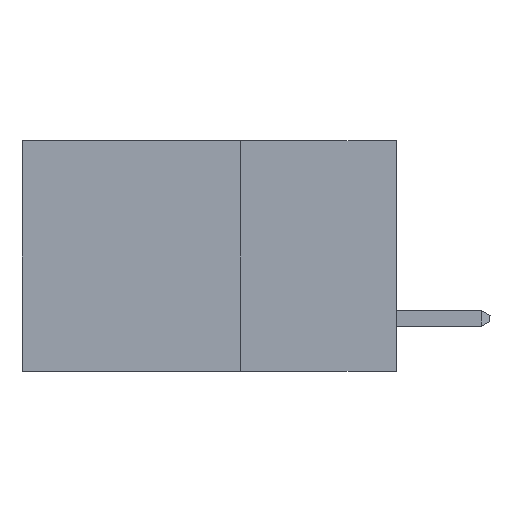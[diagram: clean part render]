
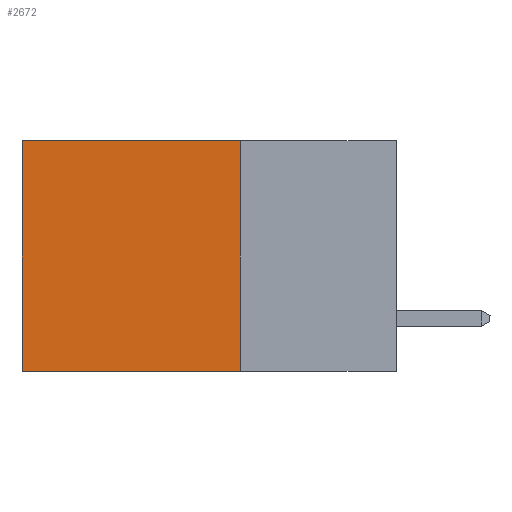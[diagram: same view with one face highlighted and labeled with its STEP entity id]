
A CAD part, left-side view. The second image highlights one B-rep face of the part: STEP entity #2672.
In plain terms, the highlighted planar face has unit normal (-1, 0, 0).
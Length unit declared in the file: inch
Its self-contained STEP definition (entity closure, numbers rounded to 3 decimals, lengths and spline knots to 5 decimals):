
#148 = EDGE_CURVE ( 'NONE', #840, #9183, #6486, .T. ) ;
#196 = CARTESIAN_POINT ( 'NONE',  ( 0.2615, 0.6, -0.37 ) ) ;
#212 = DIRECTION ( 'NONE',  ( 0., 0., -1. ) ) ;
#498 = EDGE_CURVE ( 'NONE', #6003, #9183, #7599, .T. ) ;
#619 = CARTESIAN_POINT ( 'NONE',  ( 0.2615, 0.25, 0. ) ) ;
#667 = EDGE_LOOP ( 'NONE', ( #7518, #4641, #7923, #6467 ) ) ;
#736 = CARTESIAN_POINT ( 'NONE',  ( 0.2615, 0.25, 0. ) ) ;
#840 = VERTEX_POINT ( 'NONE', #8633 ) ;
#1547 = EDGE_CURVE ( 'NONE', #11051, #840, #11816, .T. ) ;
#1702 = FACE_OUTER_BOUND ( 'NONE', #667, .T. ) ;
#1977 = VECTOR ( 'NONE', #212, 39.37008 ) ;
#2411 = VECTOR ( 'NONE', #3232, 39.37008 ) ;
#2672 = ADVANCED_FACE ( 'NONE', ( #1702 ), #12160, .F. ) ;
#2751 = DIRECTION ( 'NONE',  ( 0., 1., 0. ) ) ;
#3232 = DIRECTION ( 'NONE',  ( 0., 1., 0. ) ) ;
#3752 = CARTESIAN_POINT ( 'NONE',  ( 0.2615, 0.25, -0.37 ) ) ;
#3970 = DIRECTION ( 'NONE',  ( 0., 0., -1. ) ) ;
#4641 = ORIENTED_EDGE ( 'NONE', *, *, #148, .F. ) ;
#5104 = VECTOR ( 'NONE', #8340, 39.37008 ) ;
#5947 = AXIS2_PLACEMENT_3D ( 'NONE', #3752, #11406, #3970 ) ;
#6003 = VERTEX_POINT ( 'NONE', #6692 ) ;
#6467 = ORIENTED_EDGE ( 'NONE', *, *, #6725, .T. ) ;
#6486 = LINE ( 'NONE', #9367, #11829 ) ;
#6692 = CARTESIAN_POINT ( 'NONE',  ( 0.2615, 0.6, 0. ) ) ;
#6725 = EDGE_CURVE ( 'NONE', #11051, #6003, #11911, .T. ) ;
#7518 = ORIENTED_EDGE ( 'NONE', *, *, #498, .T. ) ;
#7599 = LINE ( 'NONE', #10456, #1977 ) ;
#7923 = ORIENTED_EDGE ( 'NONE', *, *, #1547, .F. ) ;
#8340 = DIRECTION ( 'NONE',  ( 0., 0., -1. ) ) ;
#8633 = CARTESIAN_POINT ( 'NONE',  ( 0.2615, 0.25, -0.37 ) ) ;
#9183 = VERTEX_POINT ( 'NONE', #196 ) ;
#9367 = CARTESIAN_POINT ( 'NONE',  ( 0.2615, 0.25, -0.37 ) ) ;
#10456 = CARTESIAN_POINT ( 'NONE',  ( 0.2615, 0.6, -0.37 ) ) ;
#10853 = CARTESIAN_POINT ( 'NONE',  ( 0.2615, 0.25, -0.37 ) ) ;
#11051 = VERTEX_POINT ( 'NONE', #736 ) ;
#11406 = DIRECTION ( 'NONE',  ( 1., 0., 0. ) ) ;
#11816 = LINE ( 'NONE', #10853, #5104 ) ;
#11829 = VECTOR ( 'NONE', #2751, 39.37008 ) ;
#11911 = LINE ( 'NONE', #619, #2411 ) ;
#12160 = PLANE ( 'NONE',  #5947 ) ;
